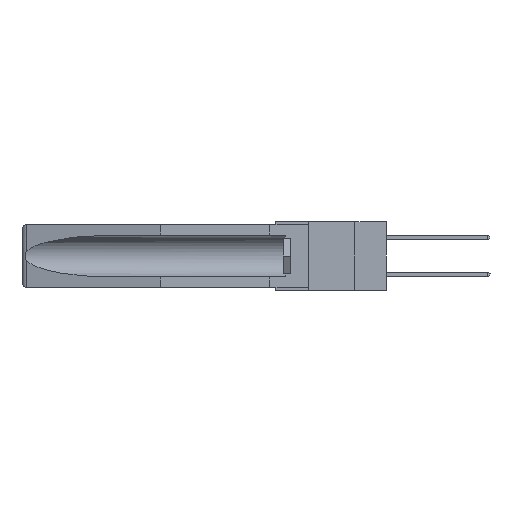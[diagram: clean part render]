
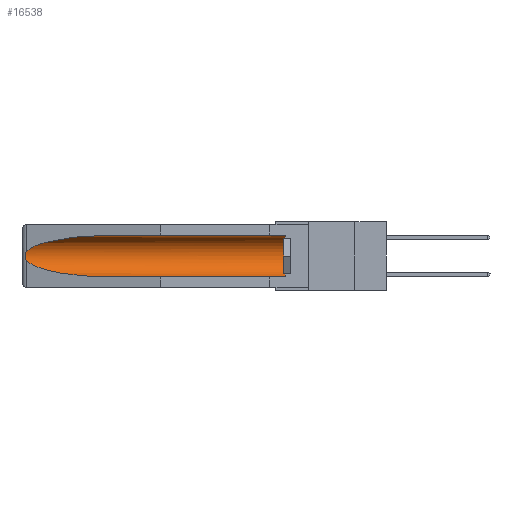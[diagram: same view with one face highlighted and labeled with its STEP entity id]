
A CAD part, left-side view. The second image highlights one B-rep face of the part: STEP entity #16538.
In plain terms, the highlighted cylindrical face has radius 2.857 mm (diameter 5.715 mm), a partial arc.
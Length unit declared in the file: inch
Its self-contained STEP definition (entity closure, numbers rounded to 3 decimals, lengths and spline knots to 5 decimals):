
#716 = CARTESIAN_POINT ( 'NONE',  ( 0.155, 1.07973, -0.284 ) ) ;
#1232 = CARTESIAN_POINT ( 'NONE',  ( 0.26537, 1.52718, -0.19328 ) ) ;
#2785 = CARTESIAN_POINT ( 'NONE',  ( 0.26597, 1.52961, -0.15275 ) ) ;
#2958 = VERTEX_POINT ( 'NONE', #10029 ) ;
#2962 = ORIENTED_EDGE ( 'NONE', *, *, #5351, .F. ) ;
#3072 = CARTESIAN_POINT ( 'NONE',  ( 0.26655, 1.53094, -0.18657 ) ) ;
#3865 = DIRECTION ( 'NONE',  ( 0., 1., 0. ) ) ;
#4994 = VERTEX_POINT ( 'NONE', #11267 ) ;
#5046 = CARTESIAN_POINT ( 'NONE',  ( 0.26654, 1.53092, -0.15636 ) ) ;
#5351 = EDGE_CURVE ( 'NONE', #2958, #27257, #15380, .T. ) ;
#5654 = CARTESIAN_POINT ( 'NONE',  ( 0.25451, 1.48313, -0.24835 ) ) ;
#5674 = ORIENTED_EDGE ( 'NONE', *, *, #25781, .T. ) ;
#6532 = CARTESIAN_POINT ( 'NONE',  ( 0.155, 0.126, -0.1715 ) ) ;
#6828 = B_SPLINE_CURVE_WITH_KNOTS ( 'NONE', 3,
 ( #15554, #2785, #5046, #26419, #17958, #19830, #24102, #3072, #7156, #9385 ),
 .UNSPECIFIED., .F., .F.,
 ( 4, 2, 2, 2, 4 ),
 ( 0., 0.00029, 0.00058, 0.00087, 0.00117 ),
 .UNSPECIFIED. ) ;
#7156 = CARTESIAN_POINT ( 'NONE',  ( 0.26597, 1.5296, -0.19026 ) ) ;
#7165 = AXIS2_PLACEMENT_3D ( 'NONE', #6532, #12925, #21351 ) ;
#7545 = EDGE_LOOP ( 'NONE', ( #5674, #25497, #17927, #2962, #19754, #23458 ) ) ;
#7564 = EDGE_CURVE ( 'NONE', #2958, #18159, #12289, .T. ) ;
#8168 = CARTESIAN_POINT ( 'NONE',  ( 0.155, -0.30754, -0.1715 ) ) ;
#8940 = CARTESIAN_POINT ( 'NONE',  ( 0.21114, 1.30732, -0.059 ) ) ;
#9385 = CARTESIAN_POINT ( 'NONE',  ( 0.26537, 1.52718, -0.19328 ) ) ;
#9764 = VECTOR ( 'NONE', #3865, 39.37008 ) ;
#10029 = CARTESIAN_POINT ( 'NONE',  ( 0.155, 0.126, -0.284 ) ) ;
#10380 = DIRECTION ( 'NONE',  ( 0., 0., 1. ) ) ;
#10965 = CARTESIAN_POINT ( 'NONE',  ( 0.155, 1.07973, -0.059 ) ) ;
#11243 = CARTESIAN_POINT ( 'NONE',  ( 0.155, 0.126, -0.059 ) ) ;
#11267 = CARTESIAN_POINT ( 'NONE',  ( 0.26537, 1.52718, -0.14972 ) ) ;
#11290 = EDGE_CURVE ( 'NONE', #23171, #27257, #11743, .T. ) ;
#11743 =( BOUNDED_CURVE ( )  B_SPLINE_CURVE ( 3, ( #13422, #5654, #26861, #716 ),
 .UNSPECIFIED., .F., .F. ) 
 B_SPLINE_CURVE_WITH_KNOTS ( ( 4, 4 ),
 ( 0.1948, 1.5708 ),
 .UNSPECIFIED. ) 
 CURVE ( )  GEOMETRIC_REPRESENTATION_ITEM ( )  RATIONAL_B_SPLINE_CURVE ( ( 1., 0.848, 0.848, 1. ) ) 
 REPRESENTATION_ITEM ( '' )  );
#12289 = CIRCLE ( 'NONE', #7165, 0.1125 ) ;
#12925 = DIRECTION ( 'NONE',  ( 0., -1., 0. ) ) ;
#13361 = CARTESIAN_POINT ( 'NONE',  ( 0.155, 1.07973, -0.059 ) ) ;
#13422 = CARTESIAN_POINT ( 'NONE',  ( 0.26537, 1.52718, -0.19328 ) ) ;
#13557 = AXIS2_PLACEMENT_3D ( 'NONE', #8168, #23252, #10380 ) ;
#13690 = EDGE_CURVE ( 'NONE', #4994, #23171, #6828, .T. ) ;
#14462 = CYLINDRICAL_SURFACE ( 'NONE', #13557, 0.1125 ) ;
#15380 = LINE ( 'NONE', #24848, #9764 ) ;
#15554 = CARTESIAN_POINT ( 'NONE',  ( 0.26537, 1.52718, -0.14972 ) ) ;
#16538 = ADVANCED_FACE ( 'NONE', ( #17417 ), #14462, .F. ) ;
#16679 = CARTESIAN_POINT ( 'NONE',  ( 0.155, 1.07973, -0.284 ) ) ;
#17417 = FACE_OUTER_BOUND ( 'NONE', #7545, .T. ) ;
#17422 = DIRECTION ( 'NONE',  ( 0., 1., 0. ) ) ;
#17927 = ORIENTED_EDGE ( 'NONE', *, *, #11290, .T. ) ;
#17958 = CARTESIAN_POINT ( 'NONE',  ( 0.2675, 1.53308, -0.16763 ) ) ;
#18009 = VERTEX_POINT ( 'NONE', #10965 ) ;
#18069 = EDGE_CURVE ( 'NONE', #18159, #18009, #20343, .T. ) ;
#18159 = VERTEX_POINT ( 'NONE', #11243 ) ;
#18675 = VECTOR ( 'NONE', #17422, 39.37008 ) ;
#19754 = ORIENTED_EDGE ( 'NONE', *, *, #7564, .T. ) ;
#19830 = CARTESIAN_POINT ( 'NONE',  ( 0.2675, 1.53308, -0.17534 ) ) ;
#20343 = LINE ( 'NONE', #21549, #18675 ) ;
#21351 = DIRECTION ( 'NONE',  ( 0., 0., 1. ) ) ;
#21431 = CARTESIAN_POINT ( 'NONE',  ( 0.26537, 1.52718, -0.14972 ) ) ;
#21523 = CARTESIAN_POINT ( 'NONE',  ( 0.25451, 1.48313, -0.09465 ) ) ;
#21549 = CARTESIAN_POINT ( 'NONE',  ( 0.155, -0.30754, -0.059 ) ) ;
#23171 = VERTEX_POINT ( 'NONE', #1232 ) ;
#23252 = DIRECTION ( 'NONE',  ( 0., 1., 0. ) ) ;
#23458 = ORIENTED_EDGE ( 'NONE', *, *, #18069, .T. ) ;
#24102 = CARTESIAN_POINT ( 'NONE',  ( 0.2673, 1.53269, -0.17917 ) ) ;
#24848 = CARTESIAN_POINT ( 'NONE',  ( 0.155, -0.30754, -0.284 ) ) ;
#25497 = ORIENTED_EDGE ( 'NONE', *, *, #13690, .T. ) ;
#25668 =( BOUNDED_CURVE ( )  B_SPLINE_CURVE ( 3, ( #13361, #8940, #21523, #21431 ),
 .UNSPECIFIED., .F., .F. ) 
 B_SPLINE_CURVE_WITH_KNOTS ( ( 4, 4 ),
 ( 4.71239, 6.08839 ),
 .UNSPECIFIED. ) 
 CURVE ( )  GEOMETRIC_REPRESENTATION_ITEM ( )  RATIONAL_B_SPLINE_CURVE ( ( 1., 0.848, 0.848, 1. ) ) 
 REPRESENTATION_ITEM ( '' )  );
#25781 = EDGE_CURVE ( 'NONE', #18009, #4994, #25668, .T. ) ;
#26419 = CARTESIAN_POINT ( 'NONE',  ( 0.2673, 1.5327, -0.16383 ) ) ;
#26861 = CARTESIAN_POINT ( 'NONE',  ( 0.21114, 1.30732, -0.284 ) ) ;
#27257 = VERTEX_POINT ( 'NONE', #16679 ) ;
